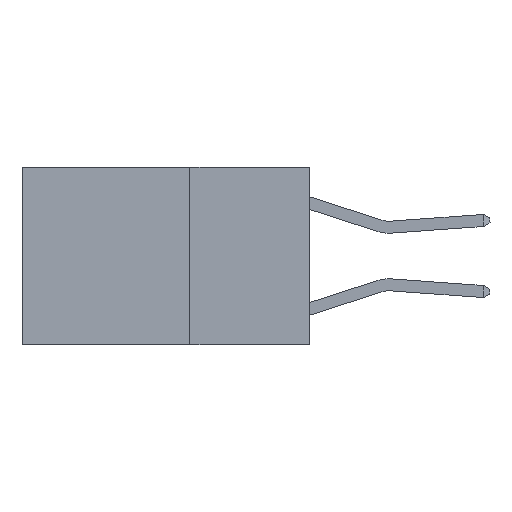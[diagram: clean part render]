
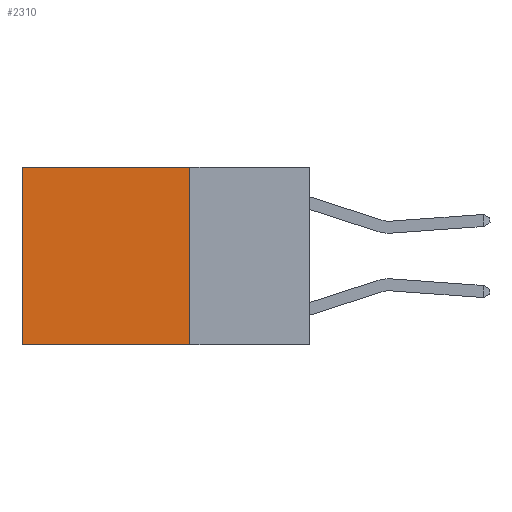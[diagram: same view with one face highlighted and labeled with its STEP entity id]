
A CAD part, left-side view. The second image highlights one B-rep face of the part: STEP entity #2310.
In plain terms, the highlighted planar face has unit normal (-1, 0, 0).
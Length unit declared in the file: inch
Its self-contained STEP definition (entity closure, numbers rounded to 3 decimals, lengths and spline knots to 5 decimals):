
#373 = DIRECTION ( 'NONE',  ( 0., 0., -1. ) ) ;
#439 = PLANE ( 'NONE',  #8614 ) ;
#908 = DIRECTION ( 'NONE',  ( 0., 1., 0. ) ) ;
#1041 = EDGE_CURVE ( 'NONE', #1914, #8077, #5454, .T. ) ;
#1082 = ORIENTED_EDGE ( 'NONE', *, *, #8134, .F. ) ;
#1446 = CARTESIAN_POINT ( 'NONE',  ( 0.2625, 0.6, -0.37 ) ) ;
#1575 = CARTESIAN_POINT ( 'NONE',  ( 0.2625, 0.25, 0. ) ) ;
#1595 = ORIENTED_EDGE ( 'NONE', *, *, #1041, .T. ) ;
#1841 = LINE ( 'NONE', #5560, #3638 ) ;
#1909 = DIRECTION ( 'NONE',  ( 0., 0., -1. ) ) ;
#1914 = VERTEX_POINT ( 'NONE', #7629 ) ;
#2164 = CARTESIAN_POINT ( 'NONE',  ( 0.2625, 0.25, -0.37 ) ) ;
#2310 = ADVANCED_FACE ( 'NONE', ( #2967 ), #439, .F. ) ;
#2618 = CARTESIAN_POINT ( 'NONE',  ( 0.2625, 0.25, 0. ) ) ;
#2967 = FACE_OUTER_BOUND ( 'NONE', #4307, .T. ) ;
#3638 = VECTOR ( 'NONE', #6971, 39.37008 ) ;
#3733 = DIRECTION ( 'NONE',  ( 0., 1., 0. ) ) ;
#3949 = EDGE_CURVE ( 'NONE', #5219, #8880, #1841, .T. ) ;
#4307 = EDGE_LOOP ( 'NONE', ( #1595, #1082, #7982, #5581 ) ) ;
#4367 = VECTOR ( 'NONE', #3733, 39.37008 ) ;
#4822 = CARTESIAN_POINT ( 'NONE',  ( 0.2625, 0.6, 0. ) ) ;
#5219 = VERTEX_POINT ( 'NONE', #2618 ) ;
#5454 = LINE ( 'NONE', #4822, #7104 ) ;
#5488 = EDGE_CURVE ( 'NONE', #5219, #1914, #6236, .T. ) ;
#5489 = CARTESIAN_POINT ( 'NONE',  ( 0.2625, 0.25, 0. ) ) ;
#5560 = CARTESIAN_POINT ( 'NONE',  ( 0.2625, 0.25, 0. ) ) ;
#5581 = ORIENTED_EDGE ( 'NONE', *, *, #5488, .T. ) ;
#6236 = LINE ( 'NONE', #1575, #4367 ) ;
#6971 = DIRECTION ( 'NONE',  ( 0., 0., -1. ) ) ;
#7104 = VECTOR ( 'NONE', #373, 39.37008 ) ;
#7432 = VECTOR ( 'NONE', #908, 39.37008 ) ;
#7629 = CARTESIAN_POINT ( 'NONE',  ( 0.2625, 0.6, 0. ) ) ;
#7730 = DIRECTION ( 'NONE',  ( 1., 0., 0. ) ) ;
#7982 = ORIENTED_EDGE ( 'NONE', *, *, #3949, .F. ) ;
#8077 = VERTEX_POINT ( 'NONE', #1446 ) ;
#8134 = EDGE_CURVE ( 'NONE', #8880, #8077, #9063, .T. ) ;
#8614 = AXIS2_PLACEMENT_3D ( 'NONE', #5489, #7730, #1909 ) ;
#8856 = CARTESIAN_POINT ( 'NONE',  ( 0.2625, 0.25, -0.37 ) ) ;
#8880 = VERTEX_POINT ( 'NONE', #8856 ) ;
#9063 = LINE ( 'NONE', #2164, #7432 ) ;
